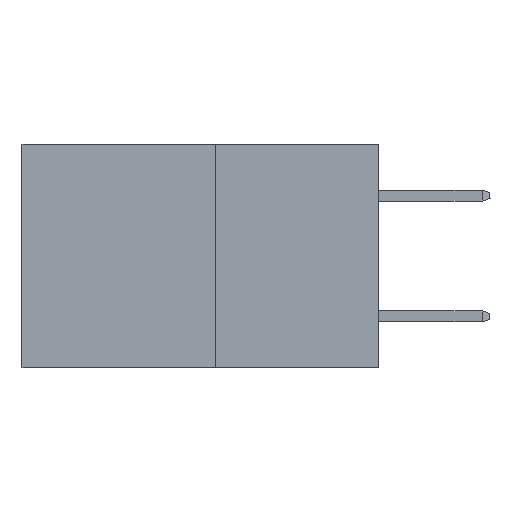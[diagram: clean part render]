
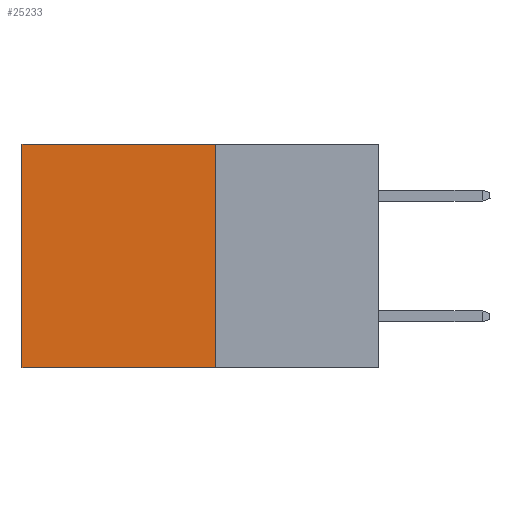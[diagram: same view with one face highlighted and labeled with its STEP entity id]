
A CAD part, left-side view. The second image highlights one B-rep face of the part: STEP entity #25233.
In plain terms, the highlighted planar face has unit normal (-1, 0, 0).
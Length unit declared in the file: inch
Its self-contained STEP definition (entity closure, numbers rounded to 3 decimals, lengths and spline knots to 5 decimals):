
#651 = VERTEX_POINT ( 'NONE', #4224 ) ;
#678 = FACE_OUTER_BOUND ( 'NONE', #12605, .T. ) ;
#1691 = LINE ( 'NONE', #16907, #18175 ) ;
#2119 = LINE ( 'NONE', #6392, #24239 ) ;
#2160 = DIRECTION ( 'NONE',  ( 0., 0., -1. ) ) ;
#2200 = CARTESIAN_POINT ( 'NONE',  ( 0.277, 0.27, 0. ) ) ;
#2591 = VERTEX_POINT ( 'NONE', #20107 ) ;
#2807 = EDGE_CURVE ( 'NONE', #2591, #22460, #22825, .T. ) ;
#3723 = CARTESIAN_POINT ( 'NONE',  ( 0.277, 0.27, -0.37 ) ) ;
#3920 = VERTEX_POINT ( 'NONE', #26948 ) ;
#4224 = CARTESIAN_POINT ( 'NONE',  ( 0.277, 0.27, -0.37 ) ) ;
#5875 = DIRECTION ( 'NONE',  ( 0., 0., -1. ) ) ;
#6267 = CARTESIAN_POINT ( 'NONE',  ( 0.277, 0.59, -0.37 ) ) ;
#6392 = CARTESIAN_POINT ( 'NONE',  ( 0.277, 0.27, -0.37 ) ) ;
#7344 = EDGE_CURVE ( 'NONE', #651, #22460, #1691, .T. ) ;
#7372 = LINE ( 'NONE', #2200, #18781 ) ;
#9308 = ORIENTED_EDGE ( 'NONE', *, *, #22809, .F. ) ;
#10149 = ORIENTED_EDGE ( 'NONE', *, *, #2807, .T. ) ;
#11537 = ORIENTED_EDGE ( 'NONE', *, *, #7344, .F. ) ;
#12605 = EDGE_LOOP ( 'NONE', ( #10149, #11537, #9308, #27274 ) ) ;
#16636 = PLANE ( 'NONE',  #24789 ) ;
#16787 = DIRECTION ( 'NONE',  ( 0., 1., 0. ) ) ;
#16907 = CARTESIAN_POINT ( 'NONE',  ( 0.277, 0.27, -0.37 ) ) ;
#17278 = DIRECTION ( 'NONE',  ( 0., 1., 0. ) ) ;
#18175 = VECTOR ( 'NONE', #16787, 39.37008 ) ;
#18490 = VECTOR ( 'NONE', #22517, 39.37008 ) ;
#18763 = DIRECTION ( 'NONE',  ( 1., 0., 0. ) ) ;
#18781 = VECTOR ( 'NONE', #17278, 39.37008 ) ;
#19578 = EDGE_CURVE ( 'NONE', #3920, #2591, #7372, .T. ) ;
#20107 = CARTESIAN_POINT ( 'NONE',  ( 0.277, 0.59, 0. ) ) ;
#20333 = CARTESIAN_POINT ( 'NONE',  ( 0.277, 0.59, -0.37 ) ) ;
#22460 = VERTEX_POINT ( 'NONE', #20333 ) ;
#22517 = DIRECTION ( 'NONE',  ( 0., 0., -1. ) ) ;
#22809 = EDGE_CURVE ( 'NONE', #3920, #651, #2119, .T. ) ;
#22825 = LINE ( 'NONE', #6267, #18490 ) ;
#24239 = VECTOR ( 'NONE', #2160, 39.37008 ) ;
#24789 = AXIS2_PLACEMENT_3D ( 'NONE', #3723, #18763, #5875 ) ;
#25233 = ADVANCED_FACE ( 'NONE', ( #678 ), #16636, .F. ) ;
#26948 = CARTESIAN_POINT ( 'NONE',  ( 0.277, 0.27, 0. ) ) ;
#27274 = ORIENTED_EDGE ( 'NONE', *, *, #19578, .T. ) ;
